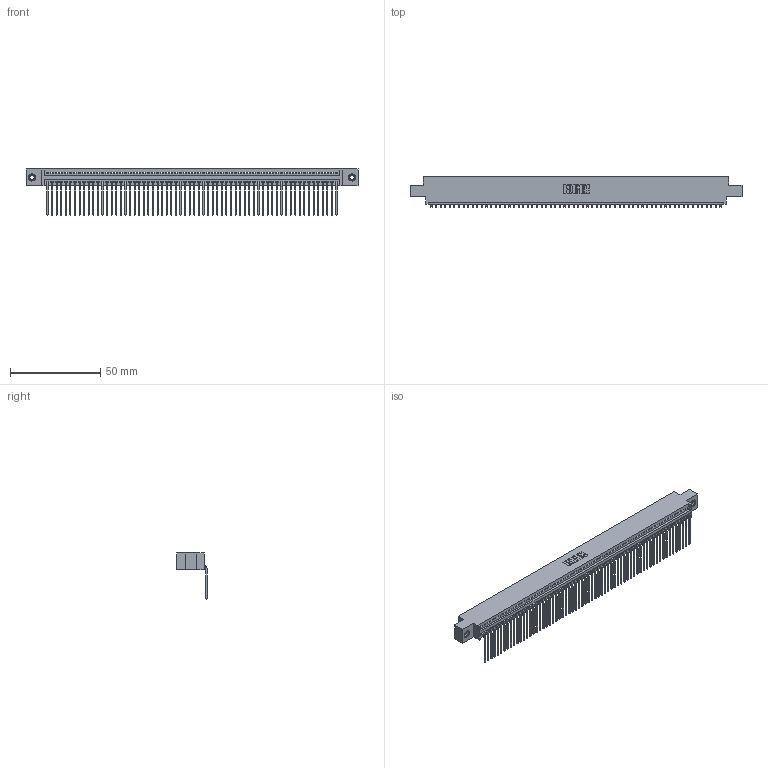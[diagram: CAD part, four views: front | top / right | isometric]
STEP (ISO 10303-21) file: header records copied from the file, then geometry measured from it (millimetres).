
FILE_DESCRIPTION (( 'STEP AP203' ), '1' );
FILE_NAME ('345-064-559-607.STEP', '2018-09-28T11:37:20', ( '' ), ( '' ), 'SwSTEP 2.0', 'SolidWorks 2016', '' );
FILE_SCHEMA (( 'CONFIG_CONTROL_DESIGN' ));
Length unit declared in the file: inch
Products named in the file (4): 345-250-001_345-250-005-103; 345-064-559-607; 345 Part_0.170 Offset - 0.156 Dia-TI; 345-292-001_558 559 Tail - 1
Assembly tree (67 placements, depth 2):
  345-064-559-607
    345 Part_0.170 Offset - 0.156 Dia-TI
    345-292-001_558 559 Tail - 1  x64
    345-250-001_345-250-005-103  x2
Bounding box: 183.77 x 16.75 x 25.53 mm (x, y, z)
Volume: 17721.1 mm3; surface area: 25260.8 mm2
Topology: 67 solids, 67 shells, 4030 faces, 12137 edges, 7998 vertices
Faces by surface type: plane 2804, cylinder 1210, cone 12, torus 4
Entity records: 46608 total; most frequent: CARTESIAN_POINT 8055, ORIENTED_EDGE 8046, DIRECTION 7029, EDGE_CURVE 4023, VECTOR 3615, LINE 3615, VERTEX_POINT 2676, AXIS2_PLACEMENT_3D 1707
